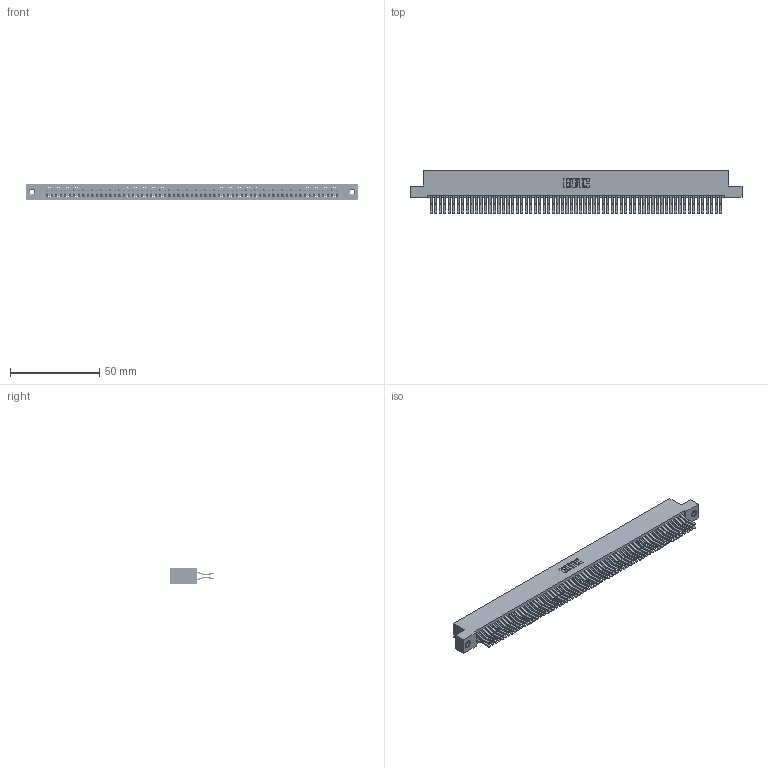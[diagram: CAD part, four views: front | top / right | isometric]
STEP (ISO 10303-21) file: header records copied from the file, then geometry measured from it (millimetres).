
FILE_DESCRIPTION (( 'STEP AP203' ), '1' );
FILE_NAME ('395-130-560-207.STEP', '2019-10-29T04:44:42', ( '' ), ( '' ), 'SwSTEP 2.0', 'SolidWorks 2016', '' );
FILE_SCHEMA (( 'CONFIG_CONTROL_DESIGN' ));
Length unit declared in the file: inch
Products named in the file (4): 345-250-001_345-250-005-103; 395-130-560-207; 345 Part_Flush Mounting Lugs - 0.156 Dia-TI; 345-292-001_560 Tail
Assembly tree (133 placements, depth 2):
  395-130-560-207
    345 Part_Flush Mounting Lugs - 0.156 Dia-TI
    345-292-001_560 Tail  x130
    345-250-001_345-250-005-103  x2
Bounding box: 186.31 x 24.45 x 9.4 mm (x, y, z)
Volume: 19150.3 mm3; surface area: 30972.2 mm2
Topology: 133 solids, 133 shells, 6946 faces, 20627 edges, 13570 vertices
Faces by surface type: plane 4402, cylinder 2528, cone 12, torus 4
Entity records: 49178 total; most frequent: CARTESIAN_POINT 8203, ORIENTED_EDGE 8130, DIRECTION 7235, EDGE_CURVE 4065, VECTOR 3649, LINE 3649, VERTEX_POINT 2704, AXIS2_PLACEMENT_3D 1793
